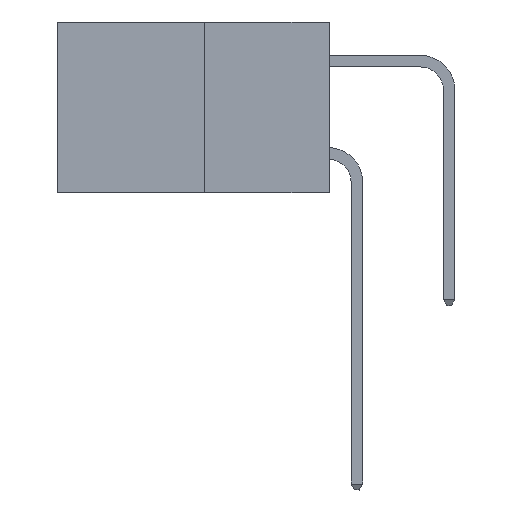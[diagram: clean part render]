
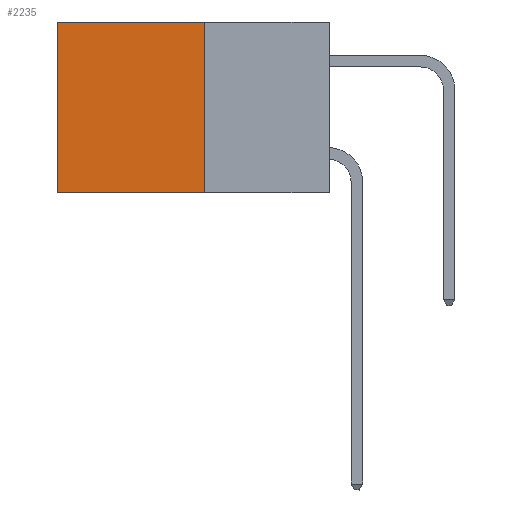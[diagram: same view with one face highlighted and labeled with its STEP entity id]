
A CAD part, left-side view. The second image highlights one B-rep face of the part: STEP entity #2235.
In plain terms, the highlighted planar face has unit normal (-1, 0, 0).
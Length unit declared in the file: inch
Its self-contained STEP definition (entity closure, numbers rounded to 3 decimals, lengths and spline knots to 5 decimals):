
#326 = EDGE_LOOP ( 'NONE', ( #5489, #3168, #8032, #954 ) ) ;
#954 = ORIENTED_EDGE ( 'NONE', *, *, #9660, .T. ) ;
#1144 = CARTESIAN_POINT ( 'NONE',  ( 0.277, 0.27, -0.37 ) ) ;
#1604 = VECTOR ( 'NONE', #9192, 39.37008 ) ;
#1614 = VERTEX_POINT ( 'NONE', #5367 ) ;
#1700 = FACE_OUTER_BOUND ( 'NONE', #326, .T. ) ;
#2057 = VECTOR ( 'NONE', #5393, 39.37008 ) ;
#2154 = CARTESIAN_POINT ( 'NONE',  ( 0.277, 0.59, -0.37 ) ) ;
#2166 = EDGE_CURVE ( 'NONE', #10307, #1614, #5342, .T. ) ;
#2235 = ADVANCED_FACE ( 'NONE', ( #1700 ), #4600, .F. ) ;
#2302 = EDGE_CURVE ( 'NONE', #8951, #8714, #10515, .T. ) ;
#3168 = ORIENTED_EDGE ( 'NONE', *, *, #9464, .F. ) ;
#3310 = VECTOR ( 'NONE', #9027, 39.37008 ) ;
#4558 = LINE ( 'NONE', #5636, #2057 ) ;
#4600 = PLANE ( 'NONE',  #10231 ) ;
#4829 = DIRECTION ( 'NONE',  ( 0., 0., -1. ) ) ;
#5045 = CARTESIAN_POINT ( 'NONE',  ( 0.277, 0.59, 0. ) ) ;
#5342 = LINE ( 'NONE', #9951, #7473 ) ;
#5367 = CARTESIAN_POINT ( 'NONE',  ( 0.277, 0.27, -0.37 ) ) ;
#5393 = DIRECTION ( 'NONE',  ( 0., 1., 0. ) ) ;
#5489 = ORIENTED_EDGE ( 'NONE', *, *, #2302, .T. ) ;
#5636 = CARTESIAN_POINT ( 'NONE',  ( 0.277, 0.27, 0. ) ) ;
#6922 = CARTESIAN_POINT ( 'NONE',  ( 0.277, 0.59, -0.37 ) ) ;
#7473 = VECTOR ( 'NONE', #8023, 39.37008 ) ;
#8023 = DIRECTION ( 'NONE',  ( 0., 0., -1. ) ) ;
#8032 = ORIENTED_EDGE ( 'NONE', *, *, #2166, .F. ) ;
#8356 = CARTESIAN_POINT ( 'NONE',  ( 0.277, 0.27, 0. ) ) ;
#8714 = VERTEX_POINT ( 'NONE', #6922 ) ;
#8951 = VERTEX_POINT ( 'NONE', #5045 ) ;
#9027 = DIRECTION ( 'NONE',  ( 0., 0., -1. ) ) ;
#9192 = DIRECTION ( 'NONE',  ( 0., 1., 0. ) ) ;
#9464 = EDGE_CURVE ( 'NONE', #1614, #8714, #10973, .T. ) ;
#9476 = CARTESIAN_POINT ( 'NONE',  ( 0.277, 0.27, -0.37 ) ) ;
#9660 = EDGE_CURVE ( 'NONE', #10307, #8951, #4558, .T. ) ;
#9916 = DIRECTION ( 'NONE',  ( 1., 0., 0. ) ) ;
#9951 = CARTESIAN_POINT ( 'NONE',  ( 0.277, 0.27, -0.37 ) ) ;
#10231 = AXIS2_PLACEMENT_3D ( 'NONE', #1144, #9916, #4829 ) ;
#10307 = VERTEX_POINT ( 'NONE', #8356 ) ;
#10515 = LINE ( 'NONE', #2154, #3310 ) ;
#10973 = LINE ( 'NONE', #9476, #1604 ) ;
